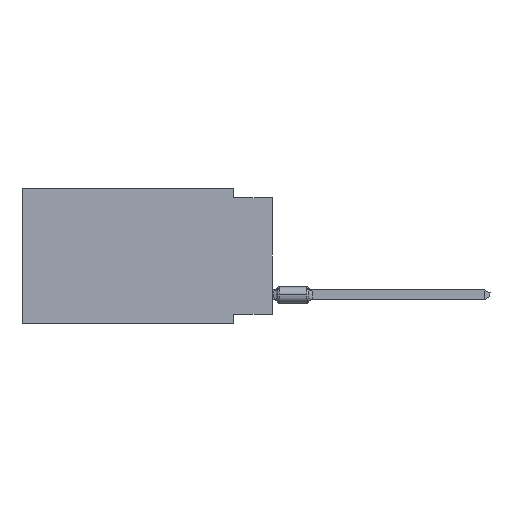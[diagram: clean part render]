
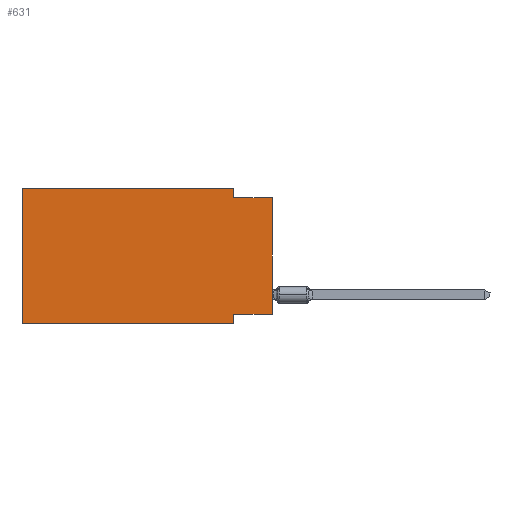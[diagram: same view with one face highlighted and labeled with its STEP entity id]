
A CAD part, left-side view. The second image highlights one B-rep face of the part: STEP entity #631.
In plain terms, the highlighted planar face has unit normal (-1, 0, 0).
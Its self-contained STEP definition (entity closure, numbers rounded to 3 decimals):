
#631 = ADVANCED_FACE ( 'NONE', ( #48888 ), #54606, .F. ) ;
#1775 = EDGE_CURVE ( 'NONE', #64215, #52705, #11971, .T. ) ;
#4749 = VERTEX_POINT ( 'NONE', #42081 ) ;
#4844 = ORIENTED_EDGE ( 'NONE', *, *, #35166, .F. ) ;
#5083 = LINE ( 'NONE', #65254, #14837 ) ;
#5896 = CARTESIAN_POINT ( 'NONE',  ( 0., 0., 0. ) ) ;
#6891 = DIRECTION ( 'NONE',  ( 0., 0., -1. ) ) ;
#7756 = VERTEX_POINT ( 'NONE', #58327 ) ;
#8665 = LINE ( 'NONE', #46998, #50965 ) ;
#8974 = ORIENTED_EDGE ( 'NONE', *, *, #36451, .F. ) ;
#11971 = LINE ( 'NONE', #5896, #15574 ) ;
#13317 = LINE ( 'NONE', #50599, #60982 ) ;
#14215 = CARTESIAN_POINT ( 'NONE',  ( 0., 0., -0.635 ) ) ;
#14570 = DIRECTION ( 'NONE',  ( 0., -1., 0. ) ) ;
#14837 = VECTOR ( 'NONE', #15473, 1000. ) ;
#15473 = DIRECTION ( 'NONE',  ( 0., -1., 0. ) ) ;
#15574 = VECTOR ( 'NONE', #65000, 1000. ) ;
#16161 = CARTESIAN_POINT ( 'NONE',  ( 0., 16.383, 0. ) ) ;
#16837 = VERTEX_POINT ( 'NONE', #26062 ) ;
#17316 = CARTESIAN_POINT ( 'NONE',  ( 0., 16.383, 0. ) ) ;
#18868 = DIRECTION ( 'NONE',  ( 0., 1., 0. ) ) ;
#21185 = DIRECTION ( 'NONE',  ( 0., 0., 1. ) ) ;
#22922 = CARTESIAN_POINT ( 'NONE',  ( 0., 2.54, 0. ) ) ;
#26062 = CARTESIAN_POINT ( 'NONE',  ( 0., 2.54, -8.255 ) ) ;
#26594 = EDGE_CURVE ( 'NONE', #7756, #42894, #8665, .T. ) ;
#27051 = VERTEX_POINT ( 'NONE', #33607 ) ;
#30855 = CARTESIAN_POINT ( 'NONE',  ( 0., 0., -0.635 ) ) ;
#33033 = EDGE_CURVE ( 'NONE', #27051, #47167, #5083, .T. ) ;
#33607 = CARTESIAN_POINT ( 'NONE',  ( 0., 16.383, 0. ) ) ;
#35166 = EDGE_CURVE ( 'NONE', #64215, #16837, #57203, .T. ) ;
#35248 = ORIENTED_EDGE ( 'NONE', *, *, #39544, .F. ) ;
#36414 = CARTESIAN_POINT ( 'NONE',  ( 0., 0., -8.255 ) ) ;
#36451 = EDGE_CURVE ( 'NONE', #4749, #52705, #51839, .T. ) ;
#38921 = ORIENTED_EDGE ( 'NONE', *, *, #54566, .F. ) ;
#38966 = ORIENTED_EDGE ( 'NONE', *, *, #1775, .T. ) ;
#39544 = EDGE_CURVE ( 'NONE', #16837, #42894, #13317, .T. ) ;
#40008 = VECTOR ( 'NONE', #18868, 1000. ) ;
#40161 = VECTOR ( 'NONE', #14570, 1000. ) ;
#40745 = CARTESIAN_POINT ( 'NONE',  ( 0., 2.54, -8.89 ) ) ;
#41470 = ORIENTED_EDGE ( 'NONE', *, *, #33033, .F. ) ;
#42081 = CARTESIAN_POINT ( 'NONE',  ( 0., 2.54, -0.635 ) ) ;
#42894 = VERTEX_POINT ( 'NONE', #40745 ) ;
#46998 = CARTESIAN_POINT ( 'NONE',  ( 0., 16.383, -8.89 ) ) ;
#47167 = VERTEX_POINT ( 'NONE', #22922 ) ;
#48888 = FACE_OUTER_BOUND ( 'NONE', #51988, .T. ) ;
#49011 = DIRECTION ( 'NONE',  ( 0., 0., -1. ) ) ;
#50418 = CARTESIAN_POINT ( 'NONE',  ( 0., 2.54, 0. ) ) ;
#50599 = CARTESIAN_POINT ( 'NONE',  ( 0., 2.54, -8.89 ) ) ;
#50965 = VECTOR ( 'NONE', #63822, 1000. ) ;
#51839 = LINE ( 'NONE', #14215, #40161 ) ;
#51988 = EDGE_LOOP ( 'NONE', ( #38966, #8974, #38921, #41470, #57102, #61946, #35248, #4844 ) ) ;
#52705 = VERTEX_POINT ( 'NONE', #30855 ) ;
#52820 = EDGE_CURVE ( 'NONE', #7756, #27051, #54491, .T. ) ;
#54491 = LINE ( 'NONE', #16161, #70334 ) ;
#54566 = EDGE_CURVE ( 'NONE', #47167, #4749, #55784, .T. ) ;
#54606 = PLANE ( 'NONE',  #69196 ) ;
#55784 = LINE ( 'NONE', #50418, #61350 ) ;
#57102 = ORIENTED_EDGE ( 'NONE', *, *, #52820, .F. ) ;
#57203 = LINE ( 'NONE', #36414, #40008 ) ;
#58327 = CARTESIAN_POINT ( 'NONE',  ( 0., 16.383, -8.89 ) ) ;
#60329 = DIRECTION ( 'NONE',  ( 1., 0., 0. ) ) ;
#60982 = VECTOR ( 'NONE', #6891, 1000. ) ;
#61350 = VECTOR ( 'NONE', #49011, 1000. ) ;
#61946 = ORIENTED_EDGE ( 'NONE', *, *, #26594, .T. ) ;
#62617 = CARTESIAN_POINT ( 'NONE',  ( 0., 0., -8.255 ) ) ;
#63822 = DIRECTION ( 'NONE',  ( 0., -1., 0. ) ) ;
#64215 = VERTEX_POINT ( 'NONE', #62617 ) ;
#64989 = DIRECTION ( 'NONE',  ( 0., 0., -1. ) ) ;
#65000 = DIRECTION ( 'NONE',  ( 0., 0., 1. ) ) ;
#65254 = CARTESIAN_POINT ( 'NONE',  ( 0., 16.383, 0. ) ) ;
#69196 = AXIS2_PLACEMENT_3D ( 'NONE', #17316, #60329, #64989 ) ;
#70334 = VECTOR ( 'NONE', #21185, 1000. ) ;
